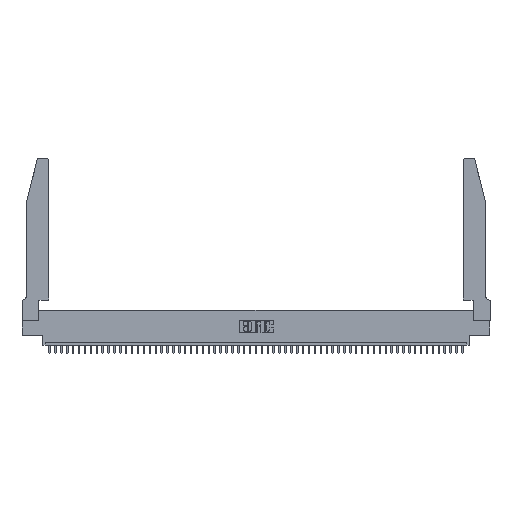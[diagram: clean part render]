
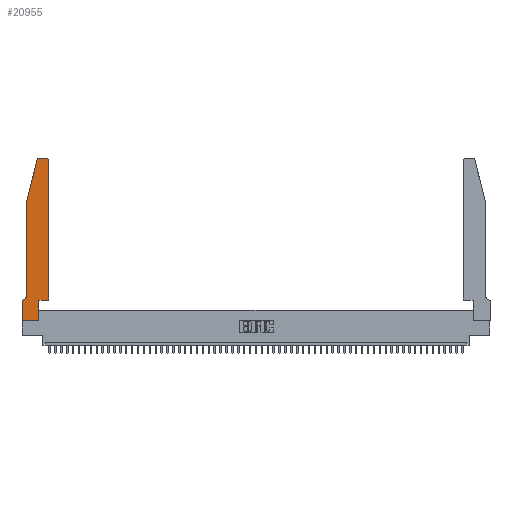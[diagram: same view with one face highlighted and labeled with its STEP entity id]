
A CAD part, top view. The second image highlights one B-rep face of the part: STEP entity #20955.
In plain terms, the highlighted planar face has unit normal (0, 0, 1).
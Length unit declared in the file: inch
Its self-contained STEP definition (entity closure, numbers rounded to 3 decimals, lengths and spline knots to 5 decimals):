
#192 = VECTOR ( 'NONE', #52602, 39.37008 ) ;
#253 = ORIENTED_EDGE ( 'NONE', *, *, #44963, .T. ) ;
#1468 = FACE_OUTER_BOUND ( 'NONE', #49648, .T. ) ;
#1843 = VECTOR ( 'NONE', #32967, 39.37008 ) ;
#2062 = EDGE_CURVE ( 'NONE', #19077, #47199, #21841, .T. ) ;
#2208 = CARTESIAN_POINT ( 'NONE',  ( 0.0755, 2., 0.37 ) ) ;
#2445 = CARTESIAN_POINT ( 'NONE',  ( 0.0755, 2., 0.37 ) ) ;
#2946 = EDGE_CURVE ( 'NONE', #12752, #22357, #42320, .T. ) ;
#3090 = DIRECTION ( 'NONE',  ( -1., 0., 0. ) ) ;
#3103 = ORIENTED_EDGE ( 'NONE', *, *, #2062, .T. ) ;
#3269 = ORIENTED_EDGE ( 'NONE', *, *, #50366, .T. ) ;
#3716 = CARTESIAN_POINT ( 'NONE',  ( 0., 0., 0.37 ) ) ;
#4214 = DIRECTION ( 'NONE',  ( 0., -1., 0. ) ) ;
#5219 = VERTEX_POINT ( 'NONE', #29317 ) ;
#5923 = CARTESIAN_POINT ( 'NONE',  ( 0.4505, 0.35, 0.37 ) ) ;
#6287 = VERTEX_POINT ( 'NONE', #19644 ) ;
#6417 = LINE ( 'NONE', #26645, #38697 ) ;
#6637 = EDGE_CURVE ( 'NONE', #5219, #46976, #20749, .T. ) ;
#6691 = VERTEX_POINT ( 'NONE', #33975 ) ;
#6832 = EDGE_CURVE ( 'NONE', #22357, #22056, #28973, .T. ) ;
#7462 = CARTESIAN_POINT ( 'NONE',  ( 0.0055, 0.35, 0.37 ) ) ;
#8493 = ORIENTED_EDGE ( 'NONE', *, *, #51541, .T. ) ;
#8969 = DIRECTION ( 'NONE',  ( 1., 0., 0. ) ) ;
#9146 = CARTESIAN_POINT ( 'NONE',  ( 0.4205, 2.72, 0.37 ) ) ;
#9430 = VERTEX_POINT ( 'NONE', #36981 ) ;
#9503 = CARTESIAN_POINT ( 'NONE',  ( 0.4505, 0.35, 0.37 ) ) ;
#9704 = CARTESIAN_POINT ( 'NONE',  ( 0., 0.35, 0.37 ) ) ;
#9882 = VECTOR ( 'NONE', #14390, 39.37008 ) ;
#10175 = DIRECTION ( 'NONE',  ( -1., 0., 0. ) ) ;
#11104 = VECTOR ( 'NONE', #48419, 39.37008 ) ;
#12346 = CARTESIAN_POINT ( 'NONE',  ( 0.0755, 0.35, 0.37 ) ) ;
#12656 = LINE ( 'NONE', #2208, #9882 ) ;
#12752 = VERTEX_POINT ( 'NONE', #39535 ) ;
#13372 = CARTESIAN_POINT ( 'NONE',  ( 0.2865, 0.35, 0.37 ) ) ;
#13990 = DIRECTION ( 'NONE',  ( 1., 0., 0. ) ) ;
#14319 = EDGE_CURVE ( 'NONE', #9430, #53257, #40493, .T. ) ;
#14390 = DIRECTION ( 'NONE',  ( 0., -1., 0. ) ) ;
#14820 = ORIENTED_EDGE ( 'NONE', *, *, #6637, .T. ) ;
#14950 = AXIS2_PLACEMENT_3D ( 'NONE', #45044, #53605, #20162 ) ;
#16407 = EDGE_CURVE ( 'NONE', #6691, #12752, #12656, .T. ) ;
#18787 = CARTESIAN_POINT ( 'NONE',  ( 0.2865, 0.35, 0.37 ) ) ;
#19077 = VERTEX_POINT ( 'NONE', #9503 ) ;
#19644 = CARTESIAN_POINT ( 'NONE',  ( 0.25487, 2.72718, 0.37 ) ) ;
#20162 = DIRECTION ( 'NONE',  ( 1., 0., 0. ) ) ;
#20197 = CARTESIAN_POINT ( 'NONE',  ( 0.0055, 0.42, 0.37 ) ) ;
#20681 = LINE ( 'NONE', #40862, #32555 ) ;
#20749 = LINE ( 'NONE', #49395, #23305 ) ;
#20955 = ADVANCED_FACE ( 'NONE', ( #1468 ), #23227, .T. ) ;
#21841 = LINE ( 'NONE', #5923, #192 ) ;
#21849 = VECTOR ( 'NONE', #23608, 39.37008 ) ;
#22056 = VERTEX_POINT ( 'NONE', #9704 ) ;
#22357 = VERTEX_POINT ( 'NONE', #7462 ) ;
#22918 = CIRCLE ( 'NONE', #39661, 0.03 ) ;
#23227 = PLANE ( 'NONE',  #28658 ) ;
#23305 = VECTOR ( 'NONE', #10175, 39.37008 ) ;
#23608 = DIRECTION ( 'NONE',  ( -0.239, -0.971, 0. ) ) ;
#26645 = CARTESIAN_POINT ( 'NONE',  ( 0.4505, 0.35, 0.37 ) ) ;
#28265 = DIRECTION ( 'NONE',  ( 1., 0., 0. ) ) ;
#28658 = AXIS2_PLACEMENT_3D ( 'NONE', #32943, #41600, #28265 ) ;
#28973 = LINE ( 'NONE', #12346, #1843 ) ;
#29317 = CARTESIAN_POINT ( 'NONE',  ( 0.4205, 2.75, 0.37 ) ) ;
#30407 = LINE ( 'NONE', #2445, #21849 ) ;
#31118 = EDGE_CURVE ( 'NONE', #22056, #9430, #20681, .T. ) ;
#31701 = EDGE_CURVE ( 'NONE', #6287, #6691, #30407, .T. ) ;
#32304 = AXIS2_PLACEMENT_3D ( 'NONE', #20197, #45625, #3090 ) ;
#32555 = VECTOR ( 'NONE', #4214, 39.37008 ) ;
#32600 = ORIENTED_EDGE ( 'NONE', *, *, #31701, .T. ) ;
#32943 = CARTESIAN_POINT ( 'NONE',  ( 0., 0.35, 0.37 ) ) ;
#32967 = DIRECTION ( 'NONE',  ( -1., 0., 0. ) ) ;
#32980 = CARTESIAN_POINT ( 'NONE',  ( 0.4505, 2.72, 0.37 ) ) ;
#33975 = CARTESIAN_POINT ( 'NONE',  ( 0.0755, 2., 0.37 ) ) ;
#34358 = ORIENTED_EDGE ( 'NONE', *, *, #14319, .T. ) ;
#35632 = ORIENTED_EDGE ( 'NONE', *, *, #6832, .T. ) ;
#36981 = CARTESIAN_POINT ( 'NONE',  ( 0., 0., 0.37 ) ) ;
#37281 = VECTOR ( 'NONE', #50197, 39.37008 ) ;
#38697 = VECTOR ( 'NONE', #13990, 39.37008 ) ;
#39045 = ORIENTED_EDGE ( 'NONE', *, *, #31118, .T. ) ;
#39535 = CARTESIAN_POINT ( 'NONE',  ( 0.0755, 0.42, 0.37 ) ) ;
#39661 = AXIS2_PLACEMENT_3D ( 'NONE', #9146, #47305, #8969 ) ;
#39869 = CIRCLE ( 'NONE', #14950, 0.03 ) ;
#40493 = LINE ( 'NONE', #3716, #37281 ) ;
#40755 = LINE ( 'NONE', #18787, #11104 ) ;
#40862 = CARTESIAN_POINT ( 'NONE',  ( 0., 0., 0.37 ) ) ;
#41600 = DIRECTION ( 'NONE',  ( 0., 0., 1. ) ) ;
#42320 = CIRCLE ( 'NONE', #32304, 0.07 ) ;
#44963 = EDGE_CURVE ( 'NONE', #46976, #6287, #39869, .T. ) ;
#45044 = CARTESIAN_POINT ( 'NONE',  ( 0.284, 2.72, 0.37 ) ) ;
#45625 = DIRECTION ( 'NONE',  ( 0., 0., -1. ) ) ;
#45812 = ORIENTED_EDGE ( 'NONE', *, *, #2946, .T. ) ;
#46224 = CARTESIAN_POINT ( 'NONE',  ( 0.2865, 0., 0.37 ) ) ;
#46750 = CARTESIAN_POINT ( 'NONE',  ( 0.284, 2.75, 0.37 ) ) ;
#46976 = VERTEX_POINT ( 'NONE', #46750 ) ;
#47199 = VERTEX_POINT ( 'NONE', #32980 ) ;
#47305 = DIRECTION ( 'NONE',  ( 0., 0., 1. ) ) ;
#48419 = DIRECTION ( 'NONE',  ( 0., 1., 0. ) ) ;
#48688 = ORIENTED_EDGE ( 'NONE', *, *, #16407, .T. ) ;
#49395 = CARTESIAN_POINT ( 'NONE',  ( 0.2605, 2.75, 0.37 ) ) ;
#49416 = EDGE_CURVE ( 'NONE', #47199, #5219, #22918, .T. ) ;
#49648 = EDGE_LOOP ( 'NONE', ( #14820, #253, #32600, #48688, #45812, #35632, #39045, #34358, #8493, #3269, #3103, #51235 ) ) ;
#50197 = DIRECTION ( 'NONE',  ( 1., 0., 0. ) ) ;
#50366 = EDGE_CURVE ( 'NONE', #51376, #19077, #6417, .T. ) ;
#51235 = ORIENTED_EDGE ( 'NONE', *, *, #49416, .T. ) ;
#51376 = VERTEX_POINT ( 'NONE', #13372 ) ;
#51541 = EDGE_CURVE ( 'NONE', #53257, #51376, #40755, .T. ) ;
#52602 = DIRECTION ( 'NONE',  ( 0., 1., 0. ) ) ;
#53257 = VERTEX_POINT ( 'NONE', #46224 ) ;
#53605 = DIRECTION ( 'NONE',  ( 0., 0., 1. ) ) ;
